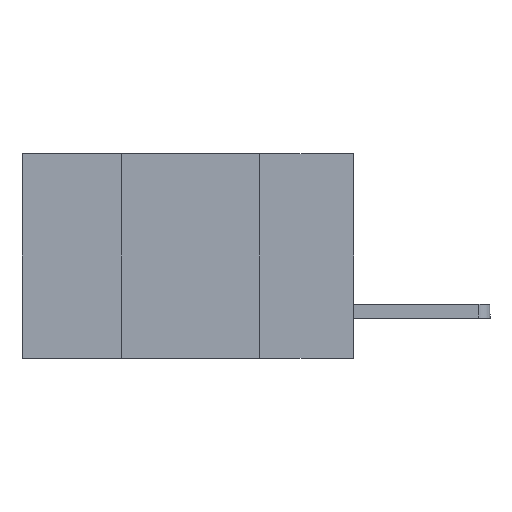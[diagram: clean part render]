
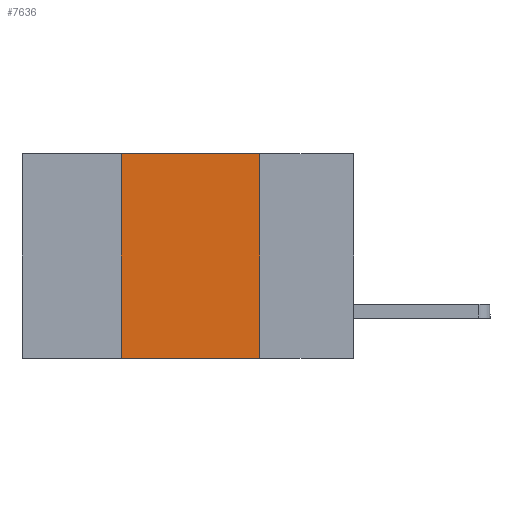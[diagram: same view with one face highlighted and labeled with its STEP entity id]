
A CAD part, left-side view. The second image highlights one B-rep face of the part: STEP entity #7636.
In plain terms, the highlighted planar face has unit normal (-1, 0, 0).
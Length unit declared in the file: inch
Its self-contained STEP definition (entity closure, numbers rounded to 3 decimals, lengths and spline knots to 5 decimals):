
#128 = CARTESIAN_POINT ( 'NONE',  ( 0., 0.17, 0. ) ) ;
#258 = VECTOR ( 'NONE', #2189, 39.37008 ) ;
#1084 = DIRECTION ( 'NONE',  ( 1., 0., 0. ) ) ;
#1284 = ORIENTED_EDGE ( 'NONE', *, *, #6297, .F. ) ;
#2189 = DIRECTION ( 'NONE',  ( 0., -1., 0. ) ) ;
#2227 = VECTOR ( 'NONE', #8821, 39.37008 ) ;
#2456 = CARTESIAN_POINT ( 'NONE',  ( 0., 0.6, -0.37 ) ) ;
#2480 = VERTEX_POINT ( 'NONE', #128 ) ;
#2704 = CARTESIAN_POINT ( 'NONE',  ( 0., 0.42, 0. ) ) ;
#2782 = VERTEX_POINT ( 'NONE', #7514 ) ;
#2819 = VERTEX_POINT ( 'NONE', #8228 ) ;
#3484 = CARTESIAN_POINT ( 'NONE',  ( 0., 0.6, 0. ) ) ;
#3790 = EDGE_CURVE ( 'NONE', #5390, #2819, #5791, .T. ) ;
#4096 = LINE ( 'NONE', #3484, #7490 ) ;
#4737 = ORIENTED_EDGE ( 'NONE', *, *, #3790, .T. ) ;
#4824 = CARTESIAN_POINT ( 'NONE',  ( 0., 0.17, 0. ) ) ;
#4974 = VECTOR ( 'NONE', #7432, 39.37008 ) ;
#5216 = CARTESIAN_POINT ( 'NONE',  ( 0., 0.6, 0. ) ) ;
#5390 = VERTEX_POINT ( 'NONE', #6458 ) ;
#5630 = ORIENTED_EDGE ( 'NONE', *, *, #6408, .F. ) ;
#5791 = LINE ( 'NONE', #2456, #258 ) ;
#5881 = PLANE ( 'NONE',  #7489 ) ;
#5913 = DIRECTION ( 'NONE',  ( 0., 0., -1. ) ) ;
#6297 = EDGE_CURVE ( 'NONE', #5390, #2782, #8525, .T. ) ;
#6303 = FACE_OUTER_BOUND ( 'NONE', #7150, .T. ) ;
#6408 = EDGE_CURVE ( 'NONE', #2782, #2480, #4096, .T. ) ;
#6458 = CARTESIAN_POINT ( 'NONE',  ( 0., 0.42, -0.37 ) ) ;
#7150 = EDGE_LOOP ( 'NONE', ( #7372, #5630, #1284, #4737 ) ) ;
#7372 = ORIENTED_EDGE ( 'NONE', *, *, #8128, .F. ) ;
#7432 = DIRECTION ( 'NONE',  ( 0., 0., 1. ) ) ;
#7489 = AXIS2_PLACEMENT_3D ( 'NONE', #5216, #1084, #5913 ) ;
#7490 = VECTOR ( 'NONE', #7562, 39.37008 ) ;
#7514 = CARTESIAN_POINT ( 'NONE',  ( 0., 0.42, 0. ) ) ;
#7562 = DIRECTION ( 'NONE',  ( 0., -1., 0. ) ) ;
#7636 = ADVANCED_FACE ( 'NONE', ( #6303 ), #5881, .F. ) ;
#7660 = LINE ( 'NONE', #4824, #2227 ) ;
#8128 = EDGE_CURVE ( 'NONE', #2480, #2819, #7660, .T. ) ;
#8228 = CARTESIAN_POINT ( 'NONE',  ( 0., 0.17, -0.37 ) ) ;
#8525 = LINE ( 'NONE', #2704, #4974 ) ;
#8821 = DIRECTION ( 'NONE',  ( 0., 0., -1. ) ) ;
